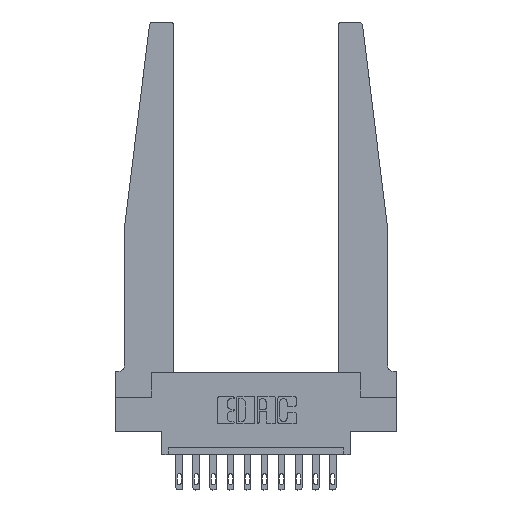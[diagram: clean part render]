
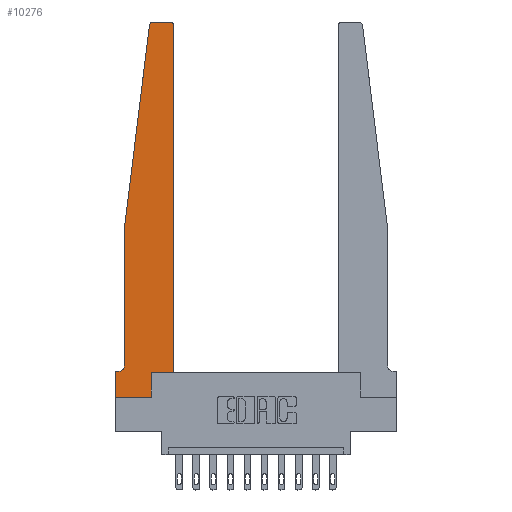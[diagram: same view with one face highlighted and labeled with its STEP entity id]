
A CAD part, top view. The second image highlights one B-rep face of the part: STEP entity #10276.
In plain terms, the highlighted planar face has unit normal (0, 0, 1).
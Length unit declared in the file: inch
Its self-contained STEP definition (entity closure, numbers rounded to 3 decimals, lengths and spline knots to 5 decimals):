
#116 = CARTESIAN_POINT ( 'NONE',  ( 0.425, 0.18, 0.37 ) ) ;
#248 = VECTOR ( 'NONE', #9823, 39.37008 ) ;
#305 = EDGE_CURVE ( 'NONE', #5915, #9452, #7764, .T. ) ;
#461 = DIRECTION ( 'NONE',  ( 0., 0., 1. ) ) ;
#562 = CARTESIAN_POINT ( 'NONE',  ( 0.065, 1.25, 0.37 ) ) ;
#656 = VERTEX_POINT ( 'NONE', #11238 ) ;
#1075 = VECTOR ( 'NONE', #6702, 39.37008 ) ;
#1087 = CARTESIAN_POINT ( 'NONE',  ( 0.065, 1.25, 0.37 ) ) ;
#1314 = EDGE_CURVE ( 'NONE', #656, #8337, #10460, .T. ) ;
#1484 = AXIS2_PLACEMENT_3D ( 'NONE', #15417, #8104, #8417 ) ;
#1554 = DIRECTION ( 'NONE',  ( 1., 0., 0. ) ) ;
#1950 = DIRECTION ( 'NONE',  ( 0., 0., -1. ) ) ;
#2023 = VECTOR ( 'NONE', #8474, 39.37008 ) ;
#2106 = CARTESIAN_POINT ( 'NONE',  ( 0.425, 0.18, 0.37 ) ) ;
#2320 = DIRECTION ( 'NONE',  ( -0.122, -0.992, 0. ) ) ;
#2392 = LINE ( 'NONE', #7287, #7296 ) ;
#2468 = ORIENTED_EDGE ( 'NONE', *, *, #2911, .T. ) ;
#2510 = AXIS2_PLACEMENT_3D ( 'NONE', #9436, #5905, #5834 ) ;
#2517 = VERTEX_POINT ( 'NONE', #5837 ) ;
#2590 = ORIENTED_EDGE ( 'NONE', *, *, #10683, .T. ) ;
#2911 = EDGE_CURVE ( 'NONE', #7622, #5915, #5351, .T. ) ;
#3272 = EDGE_CURVE ( 'NONE', #5559, #13773, #15364, .T. ) ;
#3588 = DIRECTION ( 'NONE',  ( -1., 0., 0. ) ) ;
#3671 = VECTOR ( 'NONE', #7173, 39.37008 ) ;
#3755 = CARTESIAN_POINT ( 'NONE',  ( 0.065, 0.2375, 0.37 ) ) ;
#3806 = LINE ( 'NONE', #10876, #2023 ) ;
#3809 = LINE ( 'NONE', #13504, #248 ) ;
#4420 = DIRECTION ( 'NONE',  ( 0., 1., 0. ) ) ;
#4550 = CARTESIAN_POINT ( 'NONE',  ( 0.24675, 2.72367, 0.37 ) ) ;
#4846 = EDGE_CURVE ( 'NONE', #12096, #656, #2392, .T. ) ;
#4882 = CARTESIAN_POINT ( 'NONE',  ( 0.065, 1.25, 0.37 ) ) ;
#4883 = EDGE_CURVE ( 'NONE', #8337, #7622, #6002, .T. ) ;
#5067 = ORIENTED_EDGE ( 'NONE', *, *, #6590, .T. ) ;
#5351 = LINE ( 'NONE', #562, #1075 ) ;
#5394 = ORIENTED_EDGE ( 'NONE', *, *, #11917, .T. ) ;
#5498 = EDGE_LOOP ( 'NONE', ( #14312, #8542, #14541, #2468, #10664, #10207, #5394, #12341, #2590, #14163, #9736, #5067 ) ) ;
#5559 = VERTEX_POINT ( 'NONE', #116 ) ;
#5720 = CARTESIAN_POINT ( 'NONE',  ( 0., 0.1875, 0.37 ) ) ;
#5834 = DIRECTION ( 'NONE',  ( 1., 0., 0. ) ) ;
#5837 = CARTESIAN_POINT ( 'NONE',  ( 0.2605, 0.18, 0.37 ) ) ;
#5905 = DIRECTION ( 'NONE',  ( 0., 0., 1. ) ) ;
#5915 = VERTEX_POINT ( 'NONE', #3755 ) ;
#6002 = LINE ( 'NONE', #4882, #10110 ) ;
#6017 = VERTEX_POINT ( 'NONE', #9774 ) ;
#6455 = DIRECTION ( 'NONE',  ( -1., 0., 0. ) ) ;
#6590 = EDGE_CURVE ( 'NONE', #13773, #12096, #15260, .T. ) ;
#6702 = DIRECTION ( 'NONE',  ( 0., -1., 0. ) ) ;
#6814 = CARTESIAN_POINT ( 'NONE',  ( 0.015, 0.1875, 0.37 ) ) ;
#6845 = CARTESIAN_POINT ( 'NONE',  ( 0.425, 2.72, 0.37 ) ) ;
#7089 = EDGE_CURVE ( 'NONE', #2517, #5559, #3806, .T. ) ;
#7173 = DIRECTION ( 'NONE',  ( -1., 0., 0. ) ) ;
#7287 = CARTESIAN_POINT ( 'NONE',  ( 0.25, 2.75, 0.37 ) ) ;
#7296 = VECTOR ( 'NONE', #3588, 39.37008 ) ;
#7622 = VERTEX_POINT ( 'NONE', #1087 ) ;
#7764 = CIRCLE ( 'NONE', #8275, 0.05 ) ;
#7800 = LINE ( 'NONE', #13934, #10094 ) ;
#8104 = DIRECTION ( 'NONE',  ( 0., 0., 1. ) ) ;
#8134 = CARTESIAN_POINT ( 'NONE',  ( 0.015, 0.2375, 0.37 ) ) ;
#8157 = CARTESIAN_POINT ( 'NONE',  ( 0.395, 2.75, 0.37 ) ) ;
#8275 = AXIS2_PLACEMENT_3D ( 'NONE', #8134, #1950, #6455 ) ;
#8337 = VERTEX_POINT ( 'NONE', #4550 ) ;
#8417 = DIRECTION ( 'NONE',  ( 1., 0., 0. ) ) ;
#8474 = DIRECTION ( 'NONE',  ( 1., 0., 0. ) ) ;
#8542 = ORIENTED_EDGE ( 'NONE', *, *, #1314, .T. ) ;
#9436 = CARTESIAN_POINT ( 'NONE',  ( 0.27653, 2.72, 0.37 ) ) ;
#9452 = VERTEX_POINT ( 'NONE', #6814 ) ;
#9495 = LINE ( 'NONE', #14433, #3671 ) ;
#9736 = ORIENTED_EDGE ( 'NONE', *, *, #3272, .T. ) ;
#9774 = CARTESIAN_POINT ( 'NONE',  ( 0.2605, 0., 0.37 ) ) ;
#9807 = CARTESIAN_POINT ( 'NONE',  ( 0., 0., 0.37 ) ) ;
#9823 = DIRECTION ( 'NONE',  ( 0., 1., 0. ) ) ;
#10094 = VECTOR ( 'NONE', #15052, 39.37008 ) ;
#10110 = VECTOR ( 'NONE', #2320, 39.37008 ) ;
#10150 = AXIS2_PLACEMENT_3D ( 'NONE', #12606, #461, #1554 ) ;
#10207 = ORIENTED_EDGE ( 'NONE', *, *, #12108, .T. ) ;
#10276 = ADVANCED_FACE ( 'NONE', ( #13799 ), #12534, .T. ) ;
#10460 = CIRCLE ( 'NONE', #2510, 0.03 ) ;
#10560 = VECTOR ( 'NONE', #4420, 39.37008 ) ;
#10664 = ORIENTED_EDGE ( 'NONE', *, *, #305, .T. ) ;
#10683 = EDGE_CURVE ( 'NONE', #6017, #2517, #3809, .T. ) ;
#10863 = VECTOR ( 'NONE', #13892, 39.37008 ) ;
#10876 = CARTESIAN_POINT ( 'NONE',  ( 0.425, 0.18, 0.37 ) ) ;
#11162 = VERTEX_POINT ( 'NONE', #9807 ) ;
#11238 = CARTESIAN_POINT ( 'NONE',  ( 0.27653, 2.75, 0.37 ) ) ;
#11525 = CARTESIAN_POINT ( 'NONE',  ( 0., 0., 0.37 ) ) ;
#11602 = LINE ( 'NONE', #11525, #10863 ) ;
#11917 = EDGE_CURVE ( 'NONE', #13848, #11162, #11602, .T. ) ;
#12096 = VERTEX_POINT ( 'NONE', #8157 ) ;
#12108 = EDGE_CURVE ( 'NONE', #9452, #13848, #9495, .T. ) ;
#12341 = ORIENTED_EDGE ( 'NONE', *, *, #12714, .T. ) ;
#12534 = PLANE ( 'NONE',  #10150 ) ;
#12606 = CARTESIAN_POINT ( 'NONE',  ( 0., 0.1875, 0.37 ) ) ;
#12714 = EDGE_CURVE ( 'NONE', #11162, #6017, #7800, .T. ) ;
#13504 = CARTESIAN_POINT ( 'NONE',  ( 0.2605, 0.18, 0.37 ) ) ;
#13773 = VERTEX_POINT ( 'NONE', #6845 ) ;
#13799 = FACE_OUTER_BOUND ( 'NONE', #5498, .T. ) ;
#13848 = VERTEX_POINT ( 'NONE', #5720 ) ;
#13892 = DIRECTION ( 'NONE',  ( 0., -1., 0. ) ) ;
#13934 = CARTESIAN_POINT ( 'NONE',  ( 0., 0., 0.37 ) ) ;
#14163 = ORIENTED_EDGE ( 'NONE', *, *, #7089, .T. ) ;
#14312 = ORIENTED_EDGE ( 'NONE', *, *, #4846, .T. ) ;
#14433 = CARTESIAN_POINT ( 'NONE',  ( 0.065, 0.1875, 0.37 ) ) ;
#14541 = ORIENTED_EDGE ( 'NONE', *, *, #4883, .T. ) ;
#15052 = DIRECTION ( 'NONE',  ( 1., 0., 0. ) ) ;
#15260 = CIRCLE ( 'NONE', #1484, 0.03 ) ;
#15364 = LINE ( 'NONE', #2106, #10560 ) ;
#15417 = CARTESIAN_POINT ( 'NONE',  ( 0.395, 2.72, 0.37 ) ) ;
